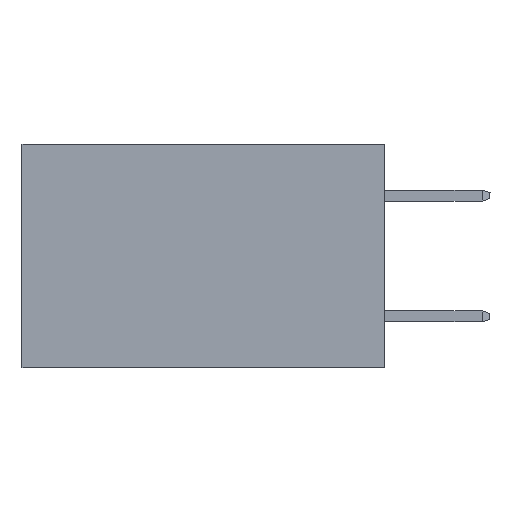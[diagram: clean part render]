
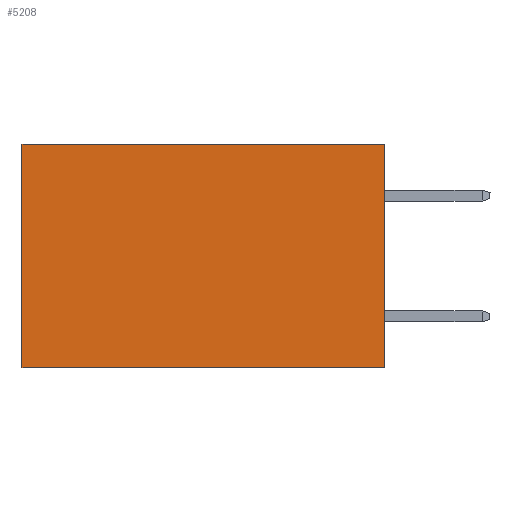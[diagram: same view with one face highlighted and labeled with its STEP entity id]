
A CAD part, left-side view. The second image highlights one B-rep face of the part: STEP entity #5208.
In plain terms, the highlighted planar face has unit normal (-1, 0, 0).
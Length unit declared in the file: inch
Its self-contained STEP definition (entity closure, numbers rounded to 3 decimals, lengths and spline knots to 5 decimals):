
#783 = VERTEX_POINT ( 'NONE', #7223 ) ;
#945 = CARTESIAN_POINT ( 'NONE',  ( 0.298, 0., 0. ) ) ;
#2447 = CARTESIAN_POINT ( 'NONE',  ( 0.298, 0., 0. ) ) ;
#2557 = VECTOR ( 'NONE', #2564, 39.37008 ) ;
#2564 = DIRECTION ( 'NONE',  ( 0., 1., 0. ) ) ;
#2814 = VECTOR ( 'NONE', #6713, 39.37008 ) ;
#3046 = AXIS2_PLACEMENT_3D ( 'NONE', #9677, #5088, #6611 ) ;
#3536 = EDGE_CURVE ( 'NONE', #7506, #7551, #8172, .T. ) ;
#3729 = EDGE_LOOP ( 'NONE', ( #8211, #3770, #9521, #6015 ) ) ;
#3770 = ORIENTED_EDGE ( 'NONE', *, *, #8237, .F. ) ;
#4056 = DIRECTION ( 'NONE',  ( 0., 1., 0. ) ) ;
#4301 = VECTOR ( 'NONE', #4056, 39.37008 ) ;
#4328 = PLANE ( 'NONE',  #3046 ) ;
#5088 = DIRECTION ( 'NONE',  ( 1., 0., 0. ) ) ;
#5208 = ADVANCED_FACE ( 'NONE', ( #6948 ), #4328, .F. ) ;
#5624 = CARTESIAN_POINT ( 'NONE',  ( 0.298, 0., -0.37 ) ) ;
#6015 = ORIENTED_EDGE ( 'NONE', *, *, #3536, .T. ) ;
#6071 = LINE ( 'NONE', #5624, #2557 ) ;
#6112 = EDGE_CURVE ( 'NONE', #7551, #6373, #7285, .T. ) ;
#6215 = DIRECTION ( 'NONE',  ( 0., 0., -1. ) ) ;
#6373 = VERTEX_POINT ( 'NONE', #8471 ) ;
#6611 = DIRECTION ( 'NONE',  ( 0., 0., -1. ) ) ;
#6713 = DIRECTION ( 'NONE',  ( 0., 0., -1. ) ) ;
#6948 = FACE_OUTER_BOUND ( 'NONE', #3729, .T. ) ;
#7223 = CARTESIAN_POINT ( 'NONE',  ( 0.298, 0., -0.37 ) ) ;
#7285 = LINE ( 'NONE', #9727, #2814 ) ;
#7506 = VERTEX_POINT ( 'NONE', #8030 ) ;
#7551 = VERTEX_POINT ( 'NONE', #9499 ) ;
#7697 = EDGE_CURVE ( 'NONE', #7506, #783, #9475, .T. ) ;
#8030 = CARTESIAN_POINT ( 'NONE',  ( 0.298, 0., 0. ) ) ;
#8172 = LINE ( 'NONE', #2447, #4301 ) ;
#8211 = ORIENTED_EDGE ( 'NONE', *, *, #6112, .T. ) ;
#8237 = EDGE_CURVE ( 'NONE', #783, #6373, #6071, .T. ) ;
#8471 = CARTESIAN_POINT ( 'NONE',  ( 0.298, 0.6, -0.37 ) ) ;
#9230 = VECTOR ( 'NONE', #6215, 39.37008 ) ;
#9475 = LINE ( 'NONE', #945, #9230 ) ;
#9499 = CARTESIAN_POINT ( 'NONE',  ( 0.298, 0.6, 0. ) ) ;
#9521 = ORIENTED_EDGE ( 'NONE', *, *, #7697, .F. ) ;
#9677 = CARTESIAN_POINT ( 'NONE',  ( 0.298, 0., 0. ) ) ;
#9727 = CARTESIAN_POINT ( 'NONE',  ( 0.298, 0.6, 0. ) ) ;
